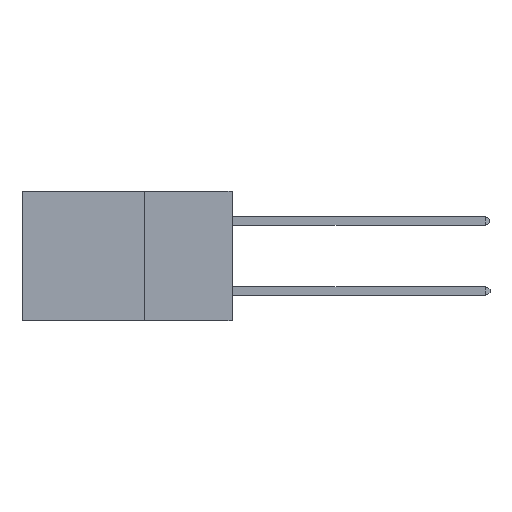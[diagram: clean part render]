
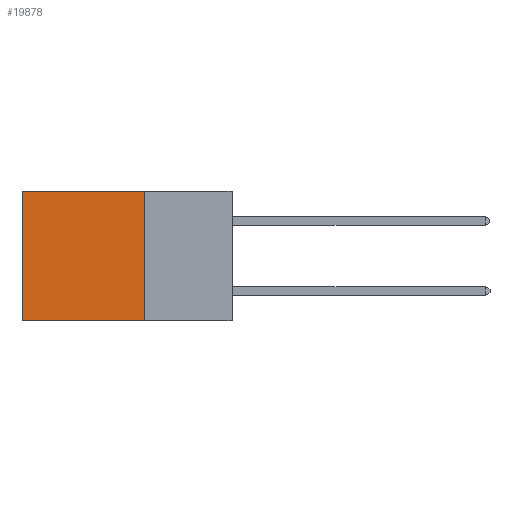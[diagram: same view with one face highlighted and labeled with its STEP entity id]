
A CAD part, left-side view. The second image highlights one B-rep face of the part: STEP entity #19878.
In plain terms, the highlighted planar face has unit normal (-1, 0, 0).
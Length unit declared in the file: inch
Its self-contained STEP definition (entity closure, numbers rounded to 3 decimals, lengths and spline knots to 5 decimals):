
#318 = DIRECTION ( 'NONE',  ( 0., 1., 0. ) ) ;
#644 = ORIENTED_EDGE ( 'NONE', *, *, #9876, .T. ) ;
#1188 = VERTEX_POINT ( 'NONE', #6838 ) ;
#1618 = VERTEX_POINT ( 'NONE', #6628 ) ;
#2048 = VECTOR ( 'NONE', #10899, 39.37008 ) ;
#3439 = EDGE_CURVE ( 'NONE', #20977, #1188, #10556, .T. ) ;
#4221 = ORIENTED_EDGE ( 'NONE', *, *, #12229, .T. ) ;
#5024 = DIRECTION ( 'NONE',  ( 1., 0., 0. ) ) ;
#5101 = VERTEX_POINT ( 'NONE', #20998 ) ;
#5468 = VECTOR ( 'NONE', #12083, 39.37008 ) ;
#6246 = VECTOR ( 'NONE', #318, 39.37008 ) ;
#6628 = CARTESIAN_POINT ( 'NONE',  ( 0.2875, 0.6, 0. ) ) ;
#6838 = CARTESIAN_POINT ( 'NONE',  ( 0.2875, 0.25, -0.37 ) ) ;
#7211 = VECTOR ( 'NONE', #8878, 39.37008 ) ;
#7776 = LINE ( 'NONE', #22702, #2048 ) ;
#8878 = DIRECTION ( 'NONE',  ( 0., 0., -1. ) ) ;
#9876 = EDGE_CURVE ( 'NONE', #20977, #1618, #14352, .T. ) ;
#10244 = CARTESIAN_POINT ( 'NONE',  ( 0.2875, 0.25, 0. ) ) ;
#10556 = LINE ( 'NONE', #10244, #5468 ) ;
#10899 = DIRECTION ( 'NONE',  ( 0., 1., 0. ) ) ;
#12083 = DIRECTION ( 'NONE',  ( 0., 0., -1. ) ) ;
#12229 = EDGE_CURVE ( 'NONE', #1618, #5101, #12275, .T. ) ;
#12275 = LINE ( 'NONE', #18670, #7211 ) ;
#13432 = CARTESIAN_POINT ( 'NONE',  ( 0.2875, 0.25, 0. ) ) ;
#14352 = LINE ( 'NONE', #19658, #6246 ) ;
#14773 = PLANE ( 'NONE',  #22713 ) ;
#15199 = DIRECTION ( 'NONE',  ( 0., 0., -1. ) ) ;
#15815 = FACE_OUTER_BOUND ( 'NONE', #15927, .T. ) ;
#15927 = EDGE_LOOP ( 'NONE', ( #4221, #19540, #18609, #644 ) ) ;
#18336 = CARTESIAN_POINT ( 'NONE',  ( 0.2875, 0.25, 0. ) ) ;
#18609 = ORIENTED_EDGE ( 'NONE', *, *, #3439, .F. ) ;
#18670 = CARTESIAN_POINT ( 'NONE',  ( 0.2875, 0.6, 0. ) ) ;
#19540 = ORIENTED_EDGE ( 'NONE', *, *, #22138, .F. ) ;
#19658 = CARTESIAN_POINT ( 'NONE',  ( 0.2875, 0.25, 0. ) ) ;
#19878 = ADVANCED_FACE ( 'NONE', ( #15815 ), #14773, .F. ) ;
#20977 = VERTEX_POINT ( 'NONE', #13432 ) ;
#20998 = CARTESIAN_POINT ( 'NONE',  ( 0.2875, 0.6, -0.37 ) ) ;
#22138 = EDGE_CURVE ( 'NONE', #1188, #5101, #7776, .T. ) ;
#22702 = CARTESIAN_POINT ( 'NONE',  ( 0.2875, 0.25, -0.37 ) ) ;
#22713 = AXIS2_PLACEMENT_3D ( 'NONE', #18336, #5024, #15199 ) ;
